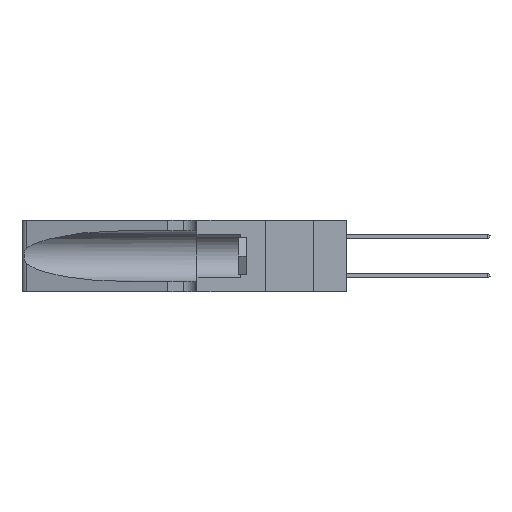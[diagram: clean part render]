
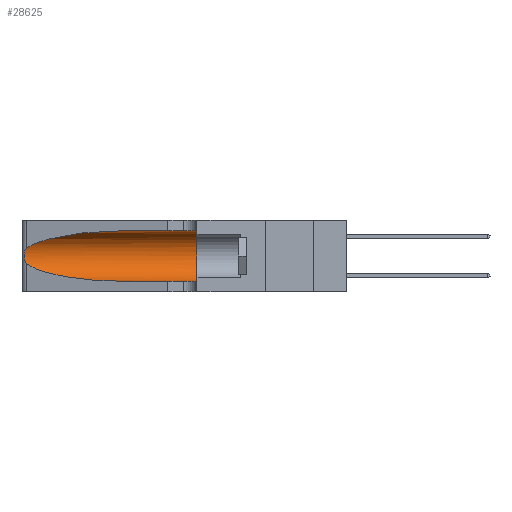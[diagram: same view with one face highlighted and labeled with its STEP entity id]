
A CAD part, left-side view. The second image highlights one B-rep face of the part: STEP entity #28625.
In plain terms, the highlighted cylindrical face has radius 3.308 mm (diameter 6.617 mm), a partial arc.
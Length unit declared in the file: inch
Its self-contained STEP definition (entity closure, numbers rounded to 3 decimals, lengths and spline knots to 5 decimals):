
#961 = DIRECTION ( 'NONE',  ( 0., 0., -1. ) ) ;
#1467 = EDGE_CURVE ( 'NONE', #8372, #8646, #19058, .T. ) ;
#1567 = CARTESIAN_POINT ( 'NONE',  ( 0.25487, 1.22718, 0.14631 ) ) ;
#2670 = VECTOR ( 'NONE', #27310, 39.37008 ) ;
#4387 = CARTESIAN_POINT ( 'NONE',  ( 0.25639, 1.23184, 0.21858 ) ) ;
#4594 = CARTESIAN_POINT ( 'NONE',  ( 0.2373, 1.15595, 0.08982 ) ) ;
#4618 = CARTESIAN_POINT ( 'NONE',  ( 0.25487, 1.22718, 0.22369 ) ) ;
#6912 = EDGE_CURVE ( 'NONE', #9676, #32305, #28428, .T. ) ;
#7152 = CARTESIAN_POINT ( 'NONE',  ( 0.1305, 1.61858, 0.05475 ) ) ;
#7158 = CARTESIAN_POINT ( 'NONE',  ( 0.25487, 1.22718, 0.14631 ) ) ;
#7290 = CARTESIAN_POINT ( 'NONE',  ( 0.25854, 1.2359, 0.20912 ) ) ;
#7500 = CARTESIAN_POINT ( 'NONE',  ( 0.18966, 0.96281, 0.05475 ) ) ;
#8372 = VERTEX_POINT ( 'NONE', #7158 ) ;
#8646 = VERTEX_POINT ( 'NONE', #33907 ) ;
#8854 = CARTESIAN_POINT ( 'NONE',  ( 0.25487, 1.22718, 0.22369 ) ) ;
#9259 = CYLINDRICAL_SURFACE ( 'NONE', #29419, 0.13025 ) ;
#9382 = CARTESIAN_POINT ( 'NONE',  ( 0.1305, 0.35, 0.05475 ) ) ;
#9430 = LINE ( 'NONE', #7152, #2670 ) ;
#9676 = VERTEX_POINT ( 'NONE', #26837 ) ;
#10178 = CARTESIAN_POINT ( 'NONE',  ( 0.26075, 1.23896, 0.19203 ) ) ;
#11111 = CARTESIAN_POINT ( 'NONE',  ( 0.1305, 0.35, 0.185 ) ) ;
#11385 = LINE ( 'NONE', #37086, #32508 ) ;
#13062 = CARTESIAN_POINT ( 'NONE',  ( 0.26017, 1.23833, 0.17102 ) ) ;
#13167 = CARTESIAN_POINT ( 'NONE',  ( 0.1305, 0.72297, 0.31525 ) ) ;
#13537 = AXIS2_PLACEMENT_3D ( 'NONE', #11111, #31241, #14001 ) ;
#14001 = DIRECTION ( 'NONE',  ( 0., 0., 1. ) ) ;
#14041 = DIRECTION ( 'NONE',  ( 0., -1., 0. ) ) ;
#15968 = CARTESIAN_POINT ( 'NONE',  ( 0.25789, 1.23486, 0.15765 ) ) ;
#16258 = B_SPLINE_CURVE_WITH_KNOTS ( 'NONE', 3,
 ( #18777, #35890, #4387, #24527, #7290, #27451, #10178, #30317, #13062, #33170, #15968, #36012, #18898, #1567 ),
 .UNSPECIFIED., .F., .F.,
 ( 4, 2, 2, 2, 2, 2, 4 ),
 ( 0., 0.00027, 0.00053, 0.00107, 0.0016, 0.00187, 0.00214 ),
 .UNSPECIFIED. ) ;
#17845 = FACE_OUTER_BOUND ( 'NONE', #25156, .T. ) ;
#18777 = CARTESIAN_POINT ( 'NONE',  ( 0.25487, 1.22718, 0.22369 ) ) ;
#18898 = CARTESIAN_POINT ( 'NONE',  ( 0.25555, 1.22993, 0.14849 ) ) ;
#19058 =( BOUNDED_CURVE ( )  B_SPLINE_CURVE ( 3, ( #24741, #4594, #7500, #27658 ),
 .UNSPECIFIED., .F., .F. ) 
 B_SPLINE_CURVE_WITH_KNOTS ( ( 4, 4 ),
 ( 3.44316, 4.71239 ),
 .UNSPECIFIED. ) 
 CURVE ( )  GEOMETRIC_REPRESENTATION_ITEM ( )  RATIONAL_B_SPLINE_CURVE ( ( 1., 0.87, 0.87, 1. ) ) 
 REPRESENTATION_ITEM ( '' )  );
#20220 =( BOUNDED_CURVE ( )  B_SPLINE_CURVE ( 3, ( #13167, #36108, #21886, #4618 ),
 .UNSPECIFIED., .F., .F. ) 
 B_SPLINE_CURVE_WITH_KNOTS ( ( 4, 4 ),
 ( 1.5708, 2.84003 ),
 .UNSPECIFIED. ) 
 CURVE ( )  GEOMETRIC_REPRESENTATION_ITEM ( )  RATIONAL_B_SPLINE_CURVE ( ( 1., 0.87, 0.87, 1. ) ) 
 REPRESENTATION_ITEM ( '' )  );
#21886 = CARTESIAN_POINT ( 'NONE',  ( 0.2373, 1.15595, 0.28018 ) ) ;
#23494 = ORIENTED_EDGE ( 'NONE', *, *, #36366, .T. ) ;
#23694 = EDGE_CURVE ( 'NONE', #27422, #8372, #16258, .T. ) ;
#24483 = VERTEX_POINT ( 'NONE', #30769 ) ;
#24527 = CARTESIAN_POINT ( 'NONE',  ( 0.25787, 1.23484, 0.2124 ) ) ;
#24741 = CARTESIAN_POINT ( 'NONE',  ( 0.25487, 1.22718, 0.14631 ) ) ;
#24891 = ORIENTED_EDGE ( 'NONE', *, *, #23694, .T. ) ;
#25156 = EDGE_LOOP ( 'NONE', ( #23494, #24891, #25968, #26542, #27342, #27452 ) ) ;
#25968 = ORIENTED_EDGE ( 'NONE', *, *, #1467, .T. ) ;
#26347 = EDGE_CURVE ( 'NONE', #8646, #32305, #9430, .T. ) ;
#26542 = ORIENTED_EDGE ( 'NONE', *, *, #26347, .T. ) ;
#26837 = CARTESIAN_POINT ( 'NONE',  ( 0.1305, 0.35, 0.31525 ) ) ;
#27310 = DIRECTION ( 'NONE',  ( 0., -1., 0. ) ) ;
#27342 = ORIENTED_EDGE ( 'NONE', *, *, #6912, .F. ) ;
#27422 = VERTEX_POINT ( 'NONE', #8854 ) ;
#27451 = CARTESIAN_POINT ( 'NONE',  ( 0.26018, 1.23835, 0.19895 ) ) ;
#27452 = ORIENTED_EDGE ( 'NONE', *, *, #36566, .F. ) ;
#27658 = CARTESIAN_POINT ( 'NONE',  ( 0.1305, 0.72297, 0.05475 ) ) ;
#28428 = CIRCLE ( 'NONE', #13537, 0.13025 ) ;
#28625 = ADVANCED_FACE ( 'NONE', ( #17845 ), #9259, .F. ) ;
#29419 = AXIS2_PLACEMENT_3D ( 'NONE', #35300, #29827, #961 ) ;
#29827 = DIRECTION ( 'NONE',  ( 0., -1., 0. ) ) ;
#30317 = CARTESIAN_POINT ( 'NONE',  ( 0.26075, 1.23896, 0.178 ) ) ;
#30769 = CARTESIAN_POINT ( 'NONE',  ( 0.1305, 0.72297, 0.31525 ) ) ;
#31241 = DIRECTION ( 'NONE',  ( 0., 1., 0. ) ) ;
#32305 = VERTEX_POINT ( 'NONE', #9382 ) ;
#32508 = VECTOR ( 'NONE', #14041, 39.37008 ) ;
#33170 = CARTESIAN_POINT ( 'NONE',  ( 0.25856, 1.23593, 0.16098 ) ) ;
#33907 = CARTESIAN_POINT ( 'NONE',  ( 0.1305, 0.72297, 0.05475 ) ) ;
#35300 = CARTESIAN_POINT ( 'NONE',  ( 0.1305, 1.61858, 0.185 ) ) ;
#35890 = CARTESIAN_POINT ( 'NONE',  ( 0.25555, 1.22994, 0.2215 ) ) ;
#36012 = CARTESIAN_POINT ( 'NONE',  ( 0.25639, 1.23186, 0.15144 ) ) ;
#36108 = CARTESIAN_POINT ( 'NONE',  ( 0.18966, 0.96281, 0.31525 ) ) ;
#36366 = EDGE_CURVE ( 'NONE', #24483, #27422, #20220, .T. ) ;
#36566 = EDGE_CURVE ( 'NONE', #24483, #9676, #11385, .T. ) ;
#37086 = CARTESIAN_POINT ( 'NONE',  ( 0.1305, 1.61858, 0.31525 ) ) ;
